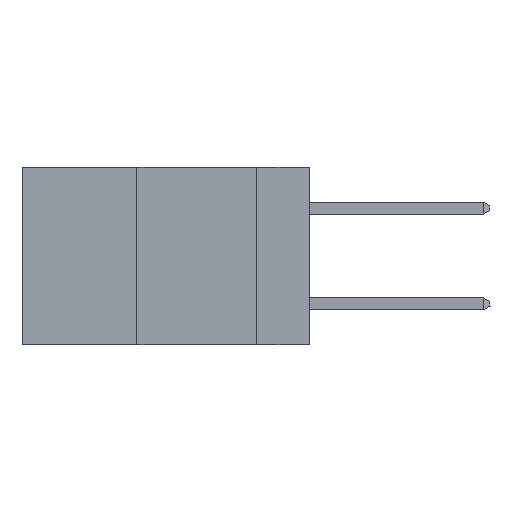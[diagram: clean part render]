
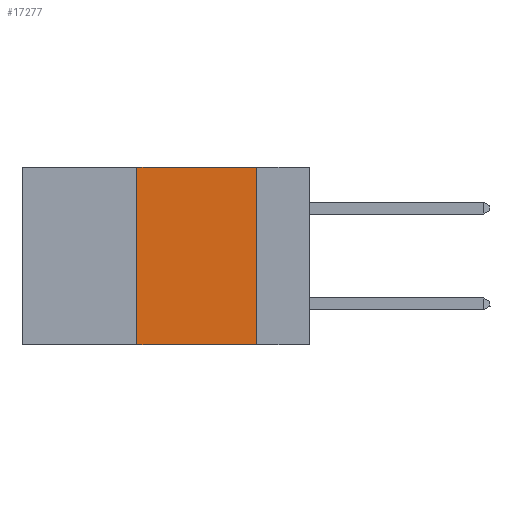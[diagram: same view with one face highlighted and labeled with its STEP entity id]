
A CAD part, left-side view. The second image highlights one B-rep face of the part: STEP entity #17277.
In plain terms, the highlighted planar face has unit normal (-1, 0, 0).
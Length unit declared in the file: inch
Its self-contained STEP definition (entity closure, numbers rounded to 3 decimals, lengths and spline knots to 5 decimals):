
#1136 = VERTEX_POINT ( 'NONE', #22564 ) ;
#2153 = EDGE_CURVE ( 'NONE', #4248, #8981, #6192, .T. ) ;
#2766 = VECTOR ( 'NONE', #21213, 39.37008 ) ;
#3023 = PLANE ( 'NONE',  #21742 ) ;
#3171 = DIRECTION ( 'NONE',  ( 1., 0., 0. ) ) ;
#3405 = CARTESIAN_POINT ( 'NONE',  ( 0., 0.11, 0. ) ) ;
#3808 = EDGE_CURVE ( 'NONE', #11329, #1136, #6392, .T. ) ;
#3994 = VECTOR ( 'NONE', #8578, 39.37008 ) ;
#4004 = DIRECTION ( 'NONE',  ( 0., -1., 0. ) ) ;
#4248 = VERTEX_POINT ( 'NONE', #26911 ) ;
#4760 = CARTESIAN_POINT ( 'NONE',  ( 0., 0.36, 0. ) ) ;
#5737 = DIRECTION ( 'NONE',  ( 0., 0., -1. ) ) ;
#6192 = LINE ( 'NONE', #16857, #21802 ) ;
#6392 = LINE ( 'NONE', #20626, #3994 ) ;
#6597 = ORIENTED_EDGE ( 'NONE', *, *, #20058, .F. ) ;
#7280 = DIRECTION ( 'NONE',  ( 0., 0., -1. ) ) ;
#8578 = DIRECTION ( 'NONE',  ( 0., -1., 0. ) ) ;
#8981 = VERTEX_POINT ( 'NONE', #24256 ) ;
#10680 = LINE ( 'NONE', #12859, #2766 ) ;
#11329 = VERTEX_POINT ( 'NONE', #4760 ) ;
#11579 = ORIENTED_EDGE ( 'NONE', *, *, #3808, .F. ) ;
#12859 = CARTESIAN_POINT ( 'NONE',  ( 0., 0.36, 0. ) ) ;
#13433 = CARTESIAN_POINT ( 'NONE',  ( 0., 0.6, 0. ) ) ;
#14222 = LINE ( 'NONE', #3405, #16592 ) ;
#16592 = VECTOR ( 'NONE', #5737, 39.37008 ) ;
#16857 = CARTESIAN_POINT ( 'NONE',  ( 0., 0.6, -0.37 ) ) ;
#17004 = EDGE_LOOP ( 'NONE', ( #6597, #11579, #18095, #21095 ) ) ;
#17277 = ADVANCED_FACE ( 'NONE', ( #19983 ), #3023, .F. ) ;
#18095 = ORIENTED_EDGE ( 'NONE', *, *, #25242, .F. ) ;
#19983 = FACE_OUTER_BOUND ( 'NONE', #17004, .T. ) ;
#20058 = EDGE_CURVE ( 'NONE', #1136, #8981, #14222, .T. ) ;
#20626 = CARTESIAN_POINT ( 'NONE',  ( 0., 0.6, 0. ) ) ;
#21095 = ORIENTED_EDGE ( 'NONE', *, *, #2153, .T. ) ;
#21213 = DIRECTION ( 'NONE',  ( 0., 0., 1. ) ) ;
#21742 = AXIS2_PLACEMENT_3D ( 'NONE', #13433, #3171, #7280 ) ;
#21802 = VECTOR ( 'NONE', #4004, 39.37008 ) ;
#22564 = CARTESIAN_POINT ( 'NONE',  ( 0., 0.11, 0. ) ) ;
#24256 = CARTESIAN_POINT ( 'NONE',  ( 0., 0.11, -0.37 ) ) ;
#25242 = EDGE_CURVE ( 'NONE', #4248, #11329, #10680, .T. ) ;
#26911 = CARTESIAN_POINT ( 'NONE',  ( 0., 0.36, -0.37 ) ) ;
